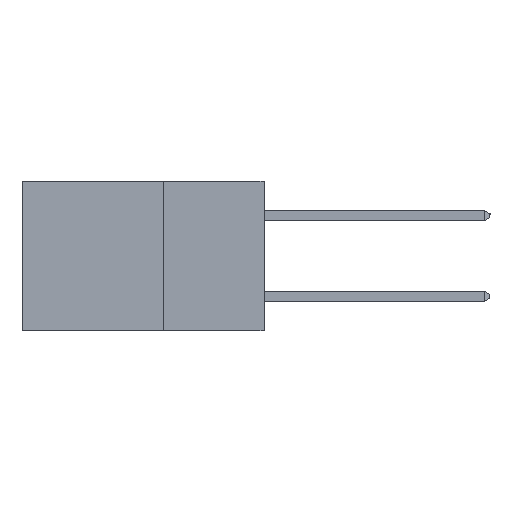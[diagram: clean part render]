
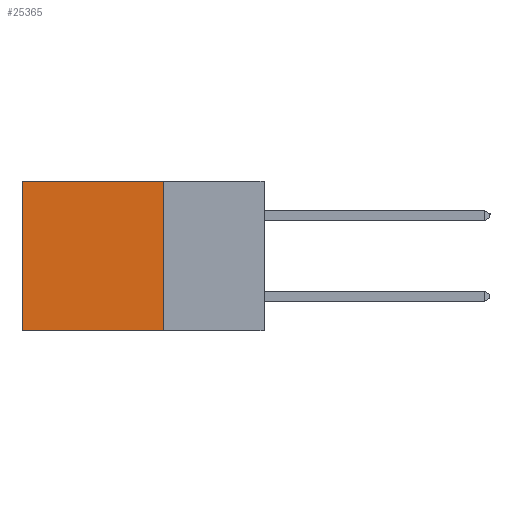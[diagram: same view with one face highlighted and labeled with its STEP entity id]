
A CAD part, left-side view. The second image highlights one B-rep face of the part: STEP entity #25365.
In plain terms, the highlighted planar face has unit normal (-1, 0, 0).
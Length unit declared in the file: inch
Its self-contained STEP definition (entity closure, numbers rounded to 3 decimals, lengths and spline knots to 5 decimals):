
#76 = DIRECTION ( 'NONE',  ( 0., 0., -1. ) ) ;
#265 = VERTEX_POINT ( 'NONE', #1073 ) ;
#555 = ORIENTED_EDGE ( 'NONE', *, *, #22411, .F. ) ;
#1073 = CARTESIAN_POINT ( 'NONE',  ( 0.2615, 0.25, -0.37 ) ) ;
#1484 = LINE ( 'NONE', #24915, #5766 ) ;
#3138 = ORIENTED_EDGE ( 'NONE', *, *, #13796, .T. ) ;
#3730 = EDGE_CURVE ( 'NONE', #15554, #265, #1484, .T. ) ;
#4257 = EDGE_CURVE ( 'NONE', #15554, #24368, #17200, .T. ) ;
#4367 = PLANE ( 'NONE',  #20508 ) ;
#4781 = CARTESIAN_POINT ( 'NONE',  ( 0.2615, 0.25, -0.37 ) ) ;
#5766 = VECTOR ( 'NONE', #21272, 39.37008 ) ;
#7459 = CARTESIAN_POINT ( 'NONE',  ( 0.2615, 0.25, 0. ) ) ;
#7907 = DIRECTION ( 'NONE',  ( 1., 0., 0. ) ) ;
#8280 = VECTOR ( 'NONE', #11463, 39.37008 ) ;
#9699 = ORIENTED_EDGE ( 'NONE', *, *, #3730, .F. ) ;
#10358 = CARTESIAN_POINT ( 'NONE',  ( 0.2615, 0.25, -0.37 ) ) ;
#10376 = LINE ( 'NONE', #4781, #14558 ) ;
#11109 = LINE ( 'NONE', #17102, #16934 ) ;
#11463 = DIRECTION ( 'NONE',  ( 0., 1., 0. ) ) ;
#13796 = EDGE_CURVE ( 'NONE', #24368, #18680, #11109, .T. ) ;
#14558 = VECTOR ( 'NONE', #22482, 39.37008 ) ;
#15276 = DIRECTION ( 'NONE',  ( 0., 0., -1. ) ) ;
#15554 = VERTEX_POINT ( 'NONE', #19158 ) ;
#16934 = VECTOR ( 'NONE', #15276, 39.37008 ) ;
#17102 = CARTESIAN_POINT ( 'NONE',  ( 0.2615, 0.6, -0.37 ) ) ;
#17200 = LINE ( 'NONE', #7459, #8280 ) ;
#17359 = CARTESIAN_POINT ( 'NONE',  ( 0.2615, 0.6, 0. ) ) ;
#17579 = ORIENTED_EDGE ( 'NONE', *, *, #4257, .T. ) ;
#17781 = FACE_OUTER_BOUND ( 'NONE', #18949, .T. ) ;
#18680 = VERTEX_POINT ( 'NONE', #23086 ) ;
#18949 = EDGE_LOOP ( 'NONE', ( #3138, #555, #9699, #17579 ) ) ;
#19158 = CARTESIAN_POINT ( 'NONE',  ( 0.2615, 0.25, 0. ) ) ;
#20508 = AXIS2_PLACEMENT_3D ( 'NONE', #10358, #7907, #76 ) ;
#21272 = DIRECTION ( 'NONE',  ( 0., 0., -1. ) ) ;
#22411 = EDGE_CURVE ( 'NONE', #265, #18680, #10376, .T. ) ;
#22482 = DIRECTION ( 'NONE',  ( 0., 1., 0. ) ) ;
#23086 = CARTESIAN_POINT ( 'NONE',  ( 0.2615, 0.6, -0.37 ) ) ;
#24368 = VERTEX_POINT ( 'NONE', #17359 ) ;
#24915 = CARTESIAN_POINT ( 'NONE',  ( 0.2615, 0.25, -0.37 ) ) ;
#25365 = ADVANCED_FACE ( 'NONE', ( #17781 ), #4367, .F. ) ;
